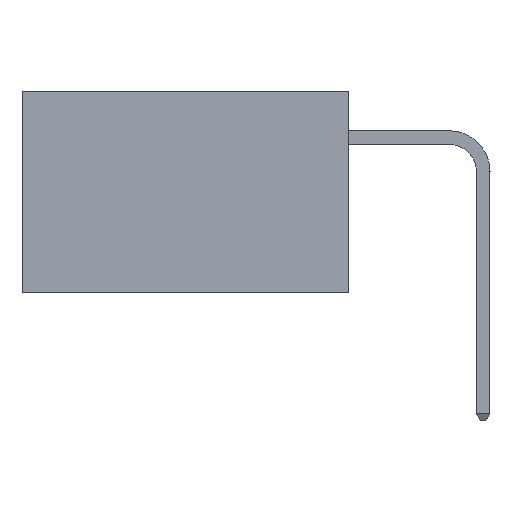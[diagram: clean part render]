
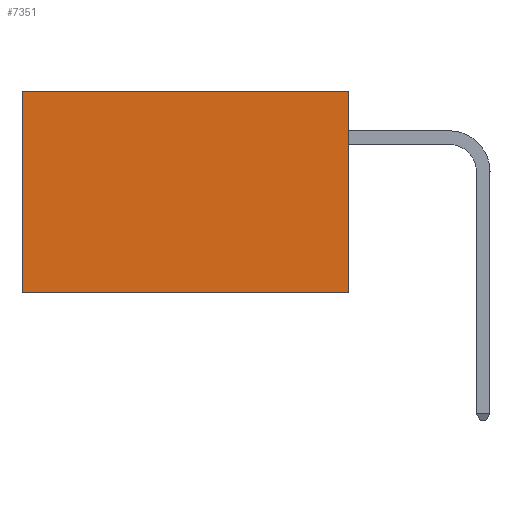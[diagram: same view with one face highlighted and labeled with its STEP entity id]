
A CAD part, left-side view. The second image highlights one B-rep face of the part: STEP entity #7351.
In plain terms, the highlighted planar face has unit normal (-1, 0, 0).
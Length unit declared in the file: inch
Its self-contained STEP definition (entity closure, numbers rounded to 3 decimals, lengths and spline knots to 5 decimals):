
#986 = PLANE ( 'NONE',  #9941 ) ;
#1109 = DIRECTION ( 'NONE',  ( 0., 0., -1. ) ) ;
#2006 = VERTEX_POINT ( 'NONE', #21091 ) ;
#2547 = DIRECTION ( 'NONE',  ( 0., 0., -1. ) ) ;
#2859 = VECTOR ( 'NONE', #25561, 39.37008 ) ;
#4337 = EDGE_CURVE ( 'NONE', #18712, #2006, #34575, .T. ) ;
#4996 = LINE ( 'NONE', #24864, #27089 ) ;
#5223 = VECTOR ( 'NONE', #17713, 39.37008 ) ;
#5780 = VERTEX_POINT ( 'NONE', #29315 ) ;
#6057 = CARTESIAN_POINT ( 'NONE',  ( 0.2875, 0., -0.37 ) ) ;
#6569 = CARTESIAN_POINT ( 'NONE',  ( 0.2875, 0., 0. ) ) ;
#6591 = ORIENTED_EDGE ( 'NONE', *, *, #29207, .F. ) ;
#7351 = ADVANCED_FACE ( 'NONE', ( #23221 ), #986, .F. ) ;
#8274 = DIRECTION ( 'NONE',  ( 0., 0., -1. ) ) ;
#8423 = VERTEX_POINT ( 'NONE', #31019 ) ;
#9323 = LINE ( 'NONE', #19277, #16719 ) ;
#9941 = AXIS2_PLACEMENT_3D ( 'NONE', #34194, #17733, #1109 ) ;
#10236 = LINE ( 'NONE', #6057, #2859 ) ;
#13729 = EDGE_CURVE ( 'NONE', #2006, #8423, #4996, .T. ) ;
#13781 = ORIENTED_EDGE ( 'NONE', *, *, #4337, .T. ) ;
#14457 = CARTESIAN_POINT ( 'NONE',  ( 0.2875, 0., 0. ) ) ;
#16719 = VECTOR ( 'NONE', #2547, 39.37008 ) ;
#17713 = DIRECTION ( 'NONE',  ( 0., 1., 0. ) ) ;
#17733 = DIRECTION ( 'NONE',  ( 1., 0., 0. ) ) ;
#18712 = VERTEX_POINT ( 'NONE', #14457 ) ;
#19277 = CARTESIAN_POINT ( 'NONE',  ( 0.2875, 0., 0. ) ) ;
#21091 = CARTESIAN_POINT ( 'NONE',  ( 0.2875, 0.6, 0. ) ) ;
#23221 = FACE_OUTER_BOUND ( 'NONE', #32824, .T. ) ;
#24864 = CARTESIAN_POINT ( 'NONE',  ( 0.2875, 0.6, 0. ) ) ;
#25561 = DIRECTION ( 'NONE',  ( 0., 1., 0. ) ) ;
#27089 = VECTOR ( 'NONE', #8274, 39.37008 ) ;
#27362 = ORIENTED_EDGE ( 'NONE', *, *, #29410, .F. ) ;
#29207 = EDGE_CURVE ( 'NONE', #18712, #5780, #9323, .T. ) ;
#29315 = CARTESIAN_POINT ( 'NONE',  ( 0.2875, 0., -0.37 ) ) ;
#29410 = EDGE_CURVE ( 'NONE', #5780, #8423, #10236, .T. ) ;
#31019 = CARTESIAN_POINT ( 'NONE',  ( 0.2875, 0.6, -0.37 ) ) ;
#31603 = ORIENTED_EDGE ( 'NONE', *, *, #13729, .T. ) ;
#32824 = EDGE_LOOP ( 'NONE', ( #31603, #27362, #6591, #13781 ) ) ;
#34194 = CARTESIAN_POINT ( 'NONE',  ( 0.2875, 0., 0. ) ) ;
#34575 = LINE ( 'NONE', #6569, #5223 ) ;
